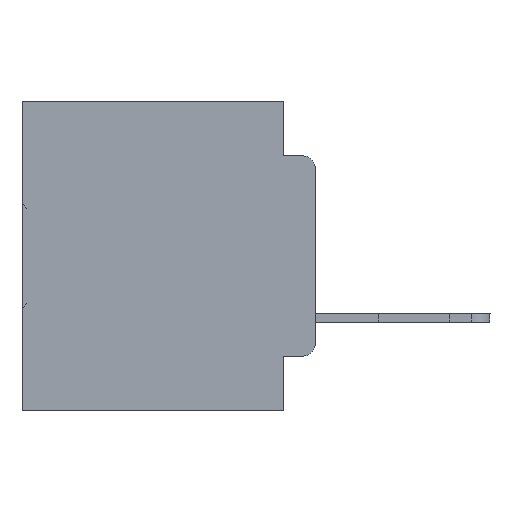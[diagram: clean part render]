
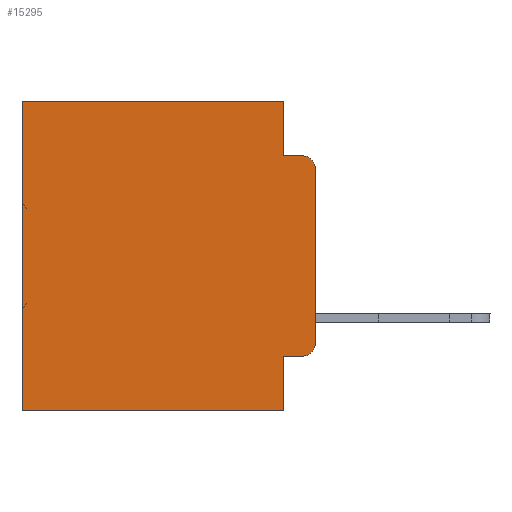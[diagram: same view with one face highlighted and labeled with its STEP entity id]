
A CAD part, left-side view. The second image highlights one B-rep face of the part: STEP entity #15295.
In plain terms, the highlighted planar face has unit normal (-1, 0, 0).
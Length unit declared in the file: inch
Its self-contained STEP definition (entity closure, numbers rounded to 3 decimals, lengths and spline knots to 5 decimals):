
#1636 = CARTESIAN_POINT ( 'NONE',  ( 0.298, 0.02, -0.4115 ) ) ;
#1870 = LINE ( 'NONE', #4385, #2429 ) ;
#1991 = VERTEX_POINT ( 'NONE', #22535 ) ;
#2429 = VECTOR ( 'NONE', #34916, 39.37008 ) ;
#2622 = LINE ( 'NONE', #18697, #25542 ) ;
#2807 = VECTOR ( 'NONE', #7847, 39.37008 ) ;
#3639 = DIRECTION ( 'NONE',  ( 0., 1., 0. ) ) ;
#3997 = CARTESIAN_POINT ( 'NONE',  ( 0.298, 0.051, -0.4115 ) ) ;
#4210 = EDGE_CURVE ( 'NONE', #14966, #18881, #9373, .T. ) ;
#4385 = CARTESIAN_POINT ( 'NONE',  ( 0.298, 0., -0.5 ) ) ;
#4950 = VECTOR ( 'NONE', #14379, 39.37008 ) ;
#5666 = EDGE_CURVE ( 'NONE', #18252, #26605, #26333, .T. ) ;
#5764 = EDGE_CURVE ( 'NONE', #12118, #1991, #29965, .T. ) ;
#6310 = CARTESIAN_POINT ( 'NONE',  ( 0.298, 0.051, -0.4115 ) ) ;
#7379 = DIRECTION ( 'NONE',  ( 0., 0., -1. ) ) ;
#7591 = CARTESIAN_POINT ( 'NONE',  ( 0.298, 0.02, -0.0885 ) ) ;
#7611 = ORIENTED_EDGE ( 'NONE', *, *, #27044, .F. ) ;
#7847 = DIRECTION ( 'NONE',  ( 0., -1., 0. ) ) ;
#9365 = ORIENTED_EDGE ( 'NONE', *, *, #33680, .T. ) ;
#9373 = LINE ( 'NONE', #6310, #19384 ) ;
#10469 = CARTESIAN_POINT ( 'NONE',  ( 0.298, 0.02, -0.1085 ) ) ;
#12007 = AXIS2_PLACEMENT_3D ( 'NONE', #21567, #35659, #27520 ) ;
#12118 = VERTEX_POINT ( 'NONE', #14870 ) ;
#14379 = DIRECTION ( 'NONE',  ( 0., 0., -1. ) ) ;
#14870 = CARTESIAN_POINT ( 'NONE',  ( 0.298, 0.051, 0. ) ) ;
#14966 = VERTEX_POINT ( 'NONE', #3997 ) ;
#15142 = EDGE_LOOP ( 'NONE', ( #7611, #33430, #26971, #22367, #20615, #15269, #22719, #30937, #33073, #9365 ) ) ;
#15269 = ORIENTED_EDGE ( 'NONE', *, *, #25640, .T. ) ;
#15285 = CARTESIAN_POINT ( 'NONE',  ( 0.298, 0., -0.1085 ) ) ;
#15295 = ADVANCED_FACE ( 'NONE', ( #27809 ), #31405, .F. ) ;
#15806 = CARTESIAN_POINT ( 'NONE',  ( 0.298, 0., 0. ) ) ;
#15972 = AXIS2_PLACEMENT_3D ( 'NONE', #10469, #23650, #7379 ) ;
#16759 = CARTESIAN_POINT ( 'NONE',  ( 0.298, 0.051, 0. ) ) ;
#17629 = VERTEX_POINT ( 'NONE', #30367 ) ;
#18252 = VERTEX_POINT ( 'NONE', #15285 ) ;
#18550 = LINE ( 'NONE', #23975, #21601 ) ;
#18665 = CARTESIAN_POINT ( 'NONE',  ( 0.298, 0.473, -0.5 ) ) ;
#18697 = CARTESIAN_POINT ( 'NONE',  ( 0.298, 0.051, 0. ) ) ;
#18881 = VERTEX_POINT ( 'NONE', #1636 ) ;
#19384 = VECTOR ( 'NONE', #20380, 39.37008 ) ;
#20263 = VERTEX_POINT ( 'NONE', #34207 ) ;
#20380 = DIRECTION ( 'NONE',  ( 0., -1., 0. ) ) ;
#20424 = LINE ( 'NONE', #23319, #32463 ) ;
#20615 = ORIENTED_EDGE ( 'NONE', *, *, #21962, .T. ) ;
#21203 = VECTOR ( 'NONE', #32850, 39.37008 ) ;
#21219 = LINE ( 'NONE', #21404, #2807 ) ;
#21404 = CARTESIAN_POINT ( 'NONE',  ( 0.298, 0.051, -0.0885 ) ) ;
#21567 = CARTESIAN_POINT ( 'NONE',  ( 0.298, 0.02, -0.3915 ) ) ;
#21601 = VECTOR ( 'NONE', #29224, 39.37008 ) ;
#21652 = EDGE_CURVE ( 'NONE', #17629, #31848, #1870, .T. ) ;
#21962 = EDGE_CURVE ( 'NONE', #12118, #20263, #20424, .T. ) ;
#22146 = CARTESIAN_POINT ( 'NONE',  ( 0.298, 0., 0. ) ) ;
#22333 = LINE ( 'NONE', #22146, #4950 ) ;
#22367 = ORIENTED_EDGE ( 'NONE', *, *, #5764, .F. ) ;
#22528 = EDGE_CURVE ( 'NONE', #14966, #17629, #2622, .T. ) ;
#22535 = CARTESIAN_POINT ( 'NONE',  ( 0.298, 0.051, -0.0885 ) ) ;
#22719 = ORIENTED_EDGE ( 'NONE', *, *, #21652, .F. ) ;
#22911 = CARTESIAN_POINT ( 'NONE',  ( 0.298, 0., -0.3915 ) ) ;
#23319 = CARTESIAN_POINT ( 'NONE',  ( 0.298, 0., 0. ) ) ;
#23650 = DIRECTION ( 'NONE',  ( -1., 0., 0. ) ) ;
#23975 = CARTESIAN_POINT ( 'NONE',  ( 0.298, 0.473, 0. ) ) ;
#25530 = VERTEX_POINT ( 'NONE', #22911 ) ;
#25542 = VECTOR ( 'NONE', #32258, 39.37008 ) ;
#25640 = EDGE_CURVE ( 'NONE', #20263, #31848, #18550, .T. ) ;
#26333 = CIRCLE ( 'NONE', #15972, 0.02 ) ;
#26605 = VERTEX_POINT ( 'NONE', #7591 ) ;
#26971 = ORIENTED_EDGE ( 'NONE', *, *, #29986, .F. ) ;
#27044 = EDGE_CURVE ( 'NONE', #18252, #25530, #22333, .T. ) ;
#27520 = DIRECTION ( 'NONE',  ( 0., 0., -1. ) ) ;
#27554 = CIRCLE ( 'NONE', #12007, 0.02 ) ;
#27809 = FACE_OUTER_BOUND ( 'NONE', #15142, .T. ) ;
#29224 = DIRECTION ( 'NONE',  ( 0., 0., -1. ) ) ;
#29913 = DIRECTION ( 'NONE',  ( 0., 0., -1. ) ) ;
#29965 = LINE ( 'NONE', #16759, #21203 ) ;
#29986 = EDGE_CURVE ( 'NONE', #1991, #26605, #21219, .T. ) ;
#30367 = CARTESIAN_POINT ( 'NONE',  ( 0.298, 0.051, -0.5 ) ) ;
#30937 = ORIENTED_EDGE ( 'NONE', *, *, #22528, .F. ) ;
#31096 = AXIS2_PLACEMENT_3D ( 'NONE', #15806, #34966, #29913 ) ;
#31405 = PLANE ( 'NONE',  #31096 ) ;
#31848 = VERTEX_POINT ( 'NONE', #18665 ) ;
#32258 = DIRECTION ( 'NONE',  ( 0., 0., -1. ) ) ;
#32463 = VECTOR ( 'NONE', #3639, 39.37008 ) ;
#32850 = DIRECTION ( 'NONE',  ( 0., 0., -1. ) ) ;
#33073 = ORIENTED_EDGE ( 'NONE', *, *, #4210, .T. ) ;
#33430 = ORIENTED_EDGE ( 'NONE', *, *, #5666, .T. ) ;
#33680 = EDGE_CURVE ( 'NONE', #18881, #25530, #27554, .T. ) ;
#34207 = CARTESIAN_POINT ( 'NONE',  ( 0.298, 0.473, 0. ) ) ;
#34916 = DIRECTION ( 'NONE',  ( 0., 1., 0. ) ) ;
#34966 = DIRECTION ( 'NONE',  ( 1., 0., 0. ) ) ;
#35659 = DIRECTION ( 'NONE',  ( -1., 0., 0. ) ) ;
